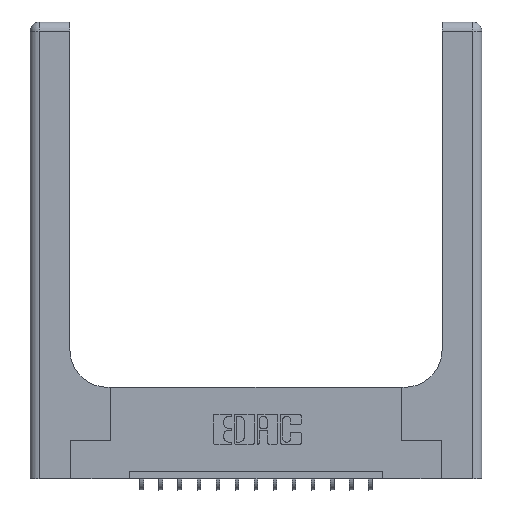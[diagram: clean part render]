
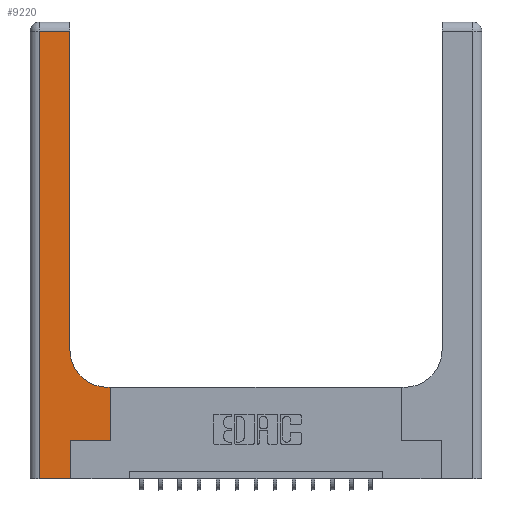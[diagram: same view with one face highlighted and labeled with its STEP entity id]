
A CAD part, top view. The second image highlights one B-rep face of the part: STEP entity #9220.
In plain terms, the highlighted planar face has unit normal (0, 0, 1).
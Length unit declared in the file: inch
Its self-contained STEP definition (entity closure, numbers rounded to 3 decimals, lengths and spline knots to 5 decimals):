
#95 = ORIENTED_EDGE ( 'NONE', *, *, #10919, .T. ) ;
#440 = DIRECTION ( 'NONE',  ( 0., 1., 0. ) ) ;
#466 = CARTESIAN_POINT ( 'NONE',  ( 0., 3., 0.37 ) ) ;
#639 = EDGE_CURVE ( 'NONE', #15017, #13844, #9273, .T. ) ;
#1073 = CARTESIAN_POINT ( 'NONE',  ( 0.26, 2.94, 0.37 ) ) ;
#1152 = CARTESIAN_POINT ( 'NONE',  ( 0.528, 0.6, 0.37 ) ) ;
#1244 = ORIENTED_EDGE ( 'NONE', *, *, #4622, .T. ) ;
#1335 = VERTEX_POINT ( 'NONE', #5496 ) ;
#1451 = CARTESIAN_POINT ( 'NONE',  ( 0.06, 3., 0.37 ) ) ;
#1843 = DIRECTION ( 'NONE',  ( -1., 0., 0. ) ) ;
#1938 = VERTEX_POINT ( 'NONE', #1073 ) ;
#2052 = VECTOR ( 'NONE', #12377, 39.37008 ) ;
#2159 = VECTOR ( 'NONE', #16143, 39.37008 ) ;
#2296 = EDGE_CURVE ( 'NONE', #16553, #1335, #7137, .T. ) ;
#2344 = VECTOR ( 'NONE', #13641, 39.37008 ) ;
#2931 = CARTESIAN_POINT ( 'NONE',  ( 0.265, 0.25, 0.37 ) ) ;
#2963 = ORIENTED_EDGE ( 'NONE', *, *, #2296, .T. ) ;
#2972 = VECTOR ( 'NONE', #440, 39.37008 ) ;
#3040 = CARTESIAN_POINT ( 'NONE',  ( 0.26, 3., 0.37 ) ) ;
#3147 = ORIENTED_EDGE ( 'NONE', *, *, #4778, .T. ) ;
#3521 = VERTEX_POINT ( 'NONE', #12065 ) ;
#3862 = EDGE_LOOP ( 'NONE', ( #3147, #10492, #16048, #2963, #14074, #1244, #13193, #95, #9473 ) ) ;
#3896 = CARTESIAN_POINT ( 'NONE',  ( 0.51, 0.85, 0.37 ) ) ;
#4579 = VERTEX_POINT ( 'NONE', #17143 ) ;
#4622 = EDGE_CURVE ( 'NONE', #12077, #15017, #11680, .T. ) ;
#4778 = EDGE_CURVE ( 'NONE', #3521, #1938, #12306, .T. ) ;
#5075 = CARTESIAN_POINT ( 'NONE',  ( 0., 2.94, 0.37 ) ) ;
#5168 = CARTESIAN_POINT ( 'NONE',  ( 0.06, 2.94, 0.37 ) ) ;
#5222 = DIRECTION ( 'NONE',  ( 1., 0., 0. ) ) ;
#5496 = CARTESIAN_POINT ( 'NONE',  ( 0.265, 0., 0.37 ) ) ;
#6140 = LINE ( 'NONE', #1451, #2159 ) ;
#6760 = LINE ( 'NONE', #12298, #2344 ) ;
#7137 = LINE ( 'NONE', #7729, #13818 ) ;
#7516 = VERTEX_POINT ( 'NONE', #5168 ) ;
#7559 = EDGE_CURVE ( 'NONE', #4579, #3521, #12711, .T. ) ;
#7729 = CARTESIAN_POINT ( 'NONE',  ( 0., 0., 0.37 ) ) ;
#7835 = VECTOR ( 'NONE', #10450, 39.37008 ) ;
#8250 = LINE ( 'NONE', #5075, #7835 ) ;
#8497 = PLANE ( 'NONE',  #9467 ) ;
#9220 = ADVANCED_FACE ( 'NONE', ( #13285 ), #8497, .F. ) ;
#9272 = CARTESIAN_POINT ( 'NONE',  ( 0.265, 0.25, 0.37 ) ) ;
#9273 = LINE ( 'NONE', #10101, #15933 ) ;
#9467 = AXIS2_PLACEMENT_3D ( 'NONE', #466, #9843, #1843 ) ;
#9473 = ORIENTED_EDGE ( 'NONE', *, *, #7559, .T. ) ;
#9843 = DIRECTION ( 'NONE',  ( 0., 0., -1. ) ) ;
#9985 = DIRECTION ( 'NONE',  ( 0., 1., 0. ) ) ;
#10056 = LINE ( 'NONE', #16413, #2972 ) ;
#10101 = CARTESIAN_POINT ( 'NONE',  ( 0.528, 0.25, 0.37 ) ) ;
#10226 = EDGE_CURVE ( 'NONE', #7516, #16553, #6140, .T. ) ;
#10228 = AXIS2_PLACEMENT_3D ( 'NONE', #3896, #13253, #5222 ) ;
#10450 = DIRECTION ( 'NONE',  ( -1., 0., 0. ) ) ;
#10492 = ORIENTED_EDGE ( 'NONE', *, *, #13815, .T. ) ;
#10919 = EDGE_CURVE ( 'NONE', #13844, #4579, #6760, .T. ) ;
#10980 = CARTESIAN_POINT ( 'NONE',  ( 0.06, 0., 0.37 ) ) ;
#11248 = VECTOR ( 'NONE', #11973, 39.37008 ) ;
#11616 = EDGE_CURVE ( 'NONE', #1335, #12077, #10056, .T. ) ;
#11680 = LINE ( 'NONE', #9272, #11248 ) ;
#11751 = DIRECTION ( 'NONE',  ( 1., 0., 0. ) ) ;
#11821 = CARTESIAN_POINT ( 'NONE',  ( 0.528, 0.25, 0.37 ) ) ;
#11973 = DIRECTION ( 'NONE',  ( 1., 0., 0. ) ) ;
#12065 = CARTESIAN_POINT ( 'NONE',  ( 0.26, 0.85, 0.37 ) ) ;
#12077 = VERTEX_POINT ( 'NONE', #2931 ) ;
#12298 = CARTESIAN_POINT ( 'NONE',  ( 0.26, 0.6, 0.37 ) ) ;
#12306 = LINE ( 'NONE', #3040, #2052 ) ;
#12377 = DIRECTION ( 'NONE',  ( 0., 1., 0. ) ) ;
#12711 = CIRCLE ( 'NONE', #10228, 0.25 ) ;
#13193 = ORIENTED_EDGE ( 'NONE', *, *, #639, .T. ) ;
#13253 = DIRECTION ( 'NONE',  ( 0., 0., -1. ) ) ;
#13285 = FACE_OUTER_BOUND ( 'NONE', #3862, .T. ) ;
#13641 = DIRECTION ( 'NONE',  ( -1., 0., 0. ) ) ;
#13815 = EDGE_CURVE ( 'NONE', #1938, #7516, #8250, .T. ) ;
#13818 = VECTOR ( 'NONE', #11751, 39.37008 ) ;
#13844 = VERTEX_POINT ( 'NONE', #1152 ) ;
#14074 = ORIENTED_EDGE ( 'NONE', *, *, #11616, .T. ) ;
#15017 = VERTEX_POINT ( 'NONE', #11821 ) ;
#15933 = VECTOR ( 'NONE', #9985, 39.37008 ) ;
#16048 = ORIENTED_EDGE ( 'NONE', *, *, #10226, .T. ) ;
#16143 = DIRECTION ( 'NONE',  ( 0., -1., 0. ) ) ;
#16413 = CARTESIAN_POINT ( 'NONE',  ( 0.265, 0., 0.37 ) ) ;
#16553 = VERTEX_POINT ( 'NONE', #10980 ) ;
#17143 = CARTESIAN_POINT ( 'NONE',  ( 0.51, 0.6, 0.37 ) ) ;
